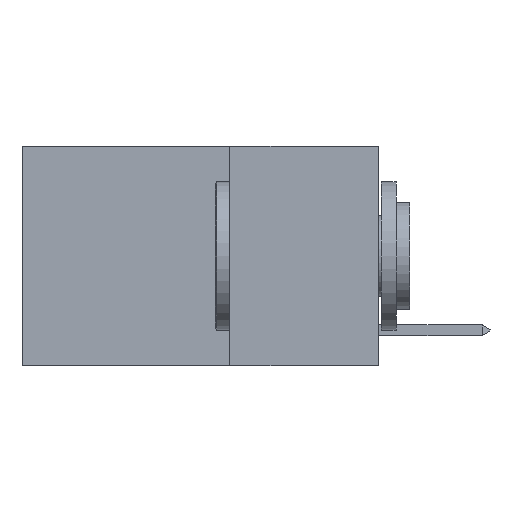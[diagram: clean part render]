
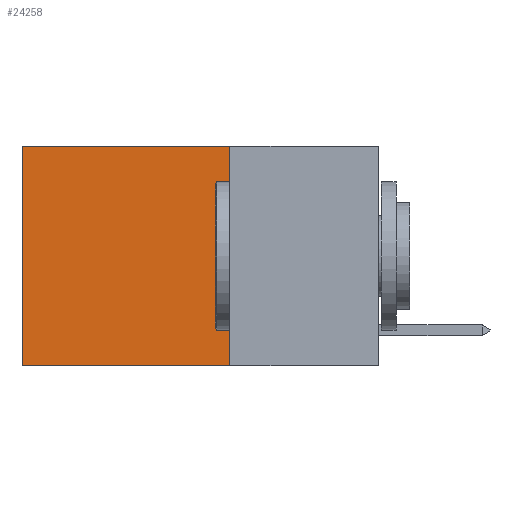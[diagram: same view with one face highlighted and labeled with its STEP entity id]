
A CAD part, left-side view. The second image highlights one B-rep face of the part: STEP entity #24258.
In plain terms, the highlighted planar face has unit normal (-1, 0, 0).
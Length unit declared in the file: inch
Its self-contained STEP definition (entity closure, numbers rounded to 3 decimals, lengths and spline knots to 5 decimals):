
#2556 = CARTESIAN_POINT ( 'NONE',  ( 0.2625, 0.25, -0.37 ) ) ;
#3161 = CARTESIAN_POINT ( 'NONE',  ( 0.2625, 0.25, 0. ) ) ;
#4107 = VECTOR ( 'NONE', #28545, 39.37008 ) ;
#5007 = LINE ( 'NONE', #2556, #15651 ) ;
#6291 = CARTESIAN_POINT ( 'NONE',  ( 0.2625, 0.25, 0. ) ) ;
#6931 = EDGE_CURVE ( 'NONE', #27656, #29012, #16240, .T. ) ;
#6969 = VECTOR ( 'NONE', #23639, 39.37008 ) ;
#7212 = CARTESIAN_POINT ( 'NONE',  ( 0.2625, 0.6, -0.37 ) ) ;
#7639 = ORIENTED_EDGE ( 'NONE', *, *, #16447, .T. ) ;
#8504 = DIRECTION ( 'NONE',  ( 0., 0., -1. ) ) ;
#9135 = LINE ( 'NONE', #25906, #6969 ) ;
#10819 = DIRECTION ( 'NONE',  ( 1., 0., 0. ) ) ;
#11248 = ORIENTED_EDGE ( 'NONE', *, *, #26517, .T. ) ;
#11984 = VERTEX_POINT ( 'NONE', #7212 ) ;
#12030 = VERTEX_POINT ( 'NONE', #25842 ) ;
#12993 = CARTESIAN_POINT ( 'NONE',  ( 0.2625, 0.25, 0. ) ) ;
#15144 = AXIS2_PLACEMENT_3D ( 'NONE', #28873, #10819, #8504 ) ;
#15651 = VECTOR ( 'NONE', #16403, 39.37008 ) ;
#16240 = LINE ( 'NONE', #12993, #4107 ) ;
#16403 = DIRECTION ( 'NONE',  ( 0., 1., 0. ) ) ;
#16447 = EDGE_CURVE ( 'NONE', #12030, #11984, #9135, .T. ) ;
#16865 = LINE ( 'NONE', #6291, #28759 ) ;
#17420 = PLANE ( 'NONE',  #15144 ) ;
#17787 = ORIENTED_EDGE ( 'NONE', *, *, #20223, .F. ) ;
#18439 = ORIENTED_EDGE ( 'NONE', *, *, #6931, .F. ) ;
#20223 = EDGE_CURVE ( 'NONE', #29012, #11984, #5007, .T. ) ;
#22241 = FACE_OUTER_BOUND ( 'NONE', #25545, .T. ) ;
#23639 = DIRECTION ( 'NONE',  ( 0., 0., -1. ) ) ;
#24258 = ADVANCED_FACE ( 'NONE', ( #22241 ), #17420, .F. ) ;
#24793 = CARTESIAN_POINT ( 'NONE',  ( 0.2625, 0.25, -0.37 ) ) ;
#25545 = EDGE_LOOP ( 'NONE', ( #7639, #17787, #18439, #11248 ) ) ;
#25842 = CARTESIAN_POINT ( 'NONE',  ( 0.2625, 0.6, 0. ) ) ;
#25906 = CARTESIAN_POINT ( 'NONE',  ( 0.2625, 0.6, 0. ) ) ;
#26517 = EDGE_CURVE ( 'NONE', #27656, #12030, #16865, .T. ) ;
#26686 = DIRECTION ( 'NONE',  ( 0., 1., 0. ) ) ;
#27656 = VERTEX_POINT ( 'NONE', #3161 ) ;
#28545 = DIRECTION ( 'NONE',  ( 0., 0., -1. ) ) ;
#28759 = VECTOR ( 'NONE', #26686, 39.37008 ) ;
#28873 = CARTESIAN_POINT ( 'NONE',  ( 0.2625, 0.25, 0. ) ) ;
#29012 = VERTEX_POINT ( 'NONE', #24793 ) ;
